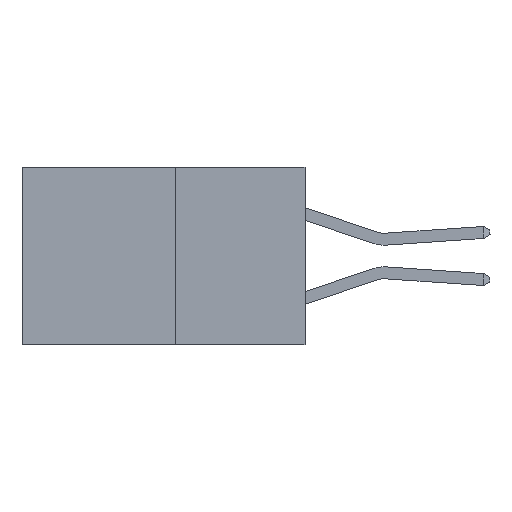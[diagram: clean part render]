
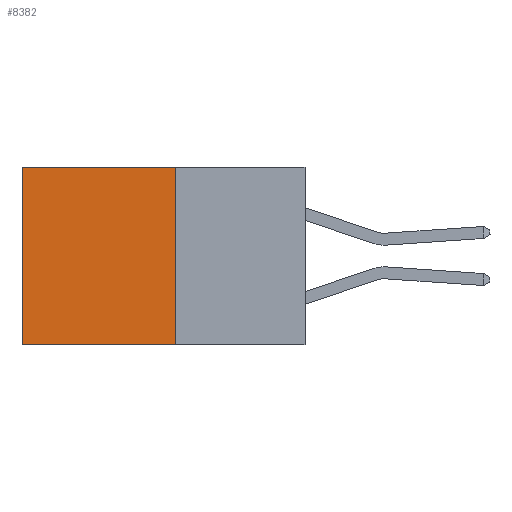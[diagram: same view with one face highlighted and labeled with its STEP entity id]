
A CAD part, left-side view. The second image highlights one B-rep face of the part: STEP entity #8382.
In plain terms, the highlighted planar face has unit normal (-1, 0, 0).
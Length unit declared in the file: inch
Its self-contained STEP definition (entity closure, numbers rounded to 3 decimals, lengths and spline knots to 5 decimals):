
#20 = EDGE_CURVE ( 'NONE', #8568, #10774, #7790, .T. ) ;
#955 = FACE_OUTER_BOUND ( 'NONE', #8801, .T. ) ;
#1935 = ORIENTED_EDGE ( 'NONE', *, *, #15261, .T. ) ;
#2447 = CARTESIAN_POINT ( 'NONE',  ( 0.277, 0.27, -0.37 ) ) ;
#2821 = CARTESIAN_POINT ( 'NONE',  ( 0.277, 0.59, 0. ) ) ;
#4121 = ORIENTED_EDGE ( 'NONE', *, *, #4472, .F. ) ;
#4472 = EDGE_CURVE ( 'NONE', #11037, #8568, #8995, .T. ) ;
#4583 = VECTOR ( 'NONE', #14969, 39.37008 ) ;
#5787 = DIRECTION ( 'NONE',  ( 1., 0., 0. ) ) ;
#6237 = LINE ( 'NONE', #8235, #11925 ) ;
#6730 = CARTESIAN_POINT ( 'NONE',  ( 0.277, 0.27, 0. ) ) ;
#7354 = AXIS2_PLACEMENT_3D ( 'NONE', #10588, #5787, #14225 ) ;
#7698 = ORIENTED_EDGE ( 'NONE', *, *, #12311, .T. ) ;
#7790 = LINE ( 'NONE', #10233, #4583 ) ;
#8076 = VERTEX_POINT ( 'NONE', #2821 ) ;
#8235 = CARTESIAN_POINT ( 'NONE',  ( 0.277, 0.59, -0.37 ) ) ;
#8382 = ADVANCED_FACE ( 'NONE', ( #955 ), #13025, .F. ) ;
#8568 = VERTEX_POINT ( 'NONE', #2447 ) ;
#8801 = EDGE_LOOP ( 'NONE', ( #1935, #12040, #4121, #7698 ) ) ;
#8995 = LINE ( 'NONE', #11693, #14985 ) ;
#10233 = CARTESIAN_POINT ( 'NONE',  ( 0.277, 0.27, -0.37 ) ) ;
#10588 = CARTESIAN_POINT ( 'NONE',  ( 0.277, 0.27, -0.37 ) ) ;
#10774 = VERTEX_POINT ( 'NONE', #11011 ) ;
#11011 = CARTESIAN_POINT ( 'NONE',  ( 0.277, 0.59, -0.37 ) ) ;
#11037 = VERTEX_POINT ( 'NONE', #6730 ) ;
#11042 = VECTOR ( 'NONE', #15046, 39.37008 ) ;
#11435 = LINE ( 'NONE', #13874, #11042 ) ;
#11693 = CARTESIAN_POINT ( 'NONE',  ( 0.277, 0.27, -0.37 ) ) ;
#11925 = VECTOR ( 'NONE', #15404, 39.37008 ) ;
#12040 = ORIENTED_EDGE ( 'NONE', *, *, #20, .F. ) ;
#12311 = EDGE_CURVE ( 'NONE', #11037, #8076, #11435, .T. ) ;
#12907 = DIRECTION ( 'NONE',  ( 0., 0., -1. ) ) ;
#13025 = PLANE ( 'NONE',  #7354 ) ;
#13874 = CARTESIAN_POINT ( 'NONE',  ( 0.277, 0.27, 0. ) ) ;
#14225 = DIRECTION ( 'NONE',  ( 0., 0., -1. ) ) ;
#14969 = DIRECTION ( 'NONE',  ( 0., 1., 0. ) ) ;
#14985 = VECTOR ( 'NONE', #12907, 39.37008 ) ;
#15046 = DIRECTION ( 'NONE',  ( 0., 1., 0. ) ) ;
#15261 = EDGE_CURVE ( 'NONE', #8076, #10774, #6237, .T. ) ;
#15404 = DIRECTION ( 'NONE',  ( 0., 0., -1. ) ) ;
